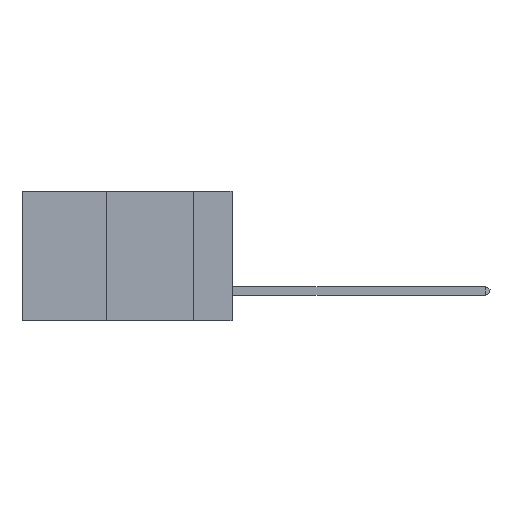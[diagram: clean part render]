
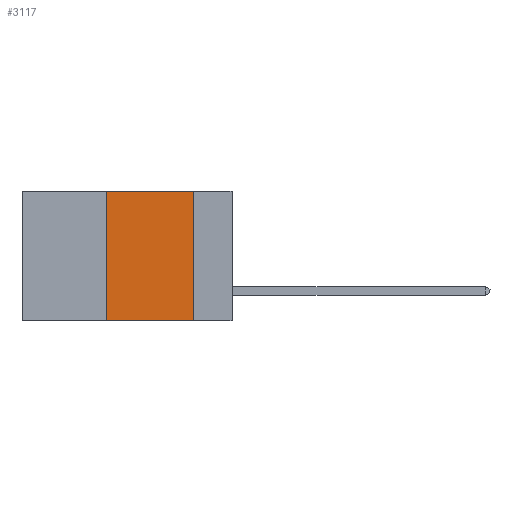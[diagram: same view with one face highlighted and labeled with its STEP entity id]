
A CAD part, left-side view. The second image highlights one B-rep face of the part: STEP entity #3117.
In plain terms, the highlighted planar face has unit normal (-1, 0, 0).
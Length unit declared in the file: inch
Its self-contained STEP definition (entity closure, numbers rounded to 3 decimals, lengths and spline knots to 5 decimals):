
#66 = DIRECTION ( 'NONE',  ( 0., -1., 0. ) ) ;
#553 = EDGE_CURVE ( 'NONE', #4618, #14399, #6563, .T. ) ;
#968 = CARTESIAN_POINT ( 'NONE',  ( 0., 0.36, 0. ) ) ;
#1084 = EDGE_CURVE ( 'NONE', #2751, #14399, #12575, .T. ) ;
#1364 = CARTESIAN_POINT ( 'NONE',  ( 0., 0.6, 0. ) ) ;
#1462 = CARTESIAN_POINT ( 'NONE',  ( 0., 0.6, -0.37 ) ) ;
#1644 = DIRECTION ( 'NONE',  ( 1., 0., 0. ) ) ;
#2654 = FACE_OUTER_BOUND ( 'NONE', #14276, .T. ) ;
#2751 = VERTEX_POINT ( 'NONE', #8409 ) ;
#2947 = ORIENTED_EDGE ( 'NONE', *, *, #553, .T. ) ;
#3117 = ADVANCED_FACE ( 'NONE', ( #2654 ), #6503, .F. ) ;
#3161 = LINE ( 'NONE', #10988, #12844 ) ;
#3299 = ORIENTED_EDGE ( 'NONE', *, *, #1084, .F. ) ;
#4618 = VERTEX_POINT ( 'NONE', #5205 ) ;
#4930 = AXIS2_PLACEMENT_3D ( 'NONE', #5303, #1644, #13589 ) ;
#5205 = CARTESIAN_POINT ( 'NONE',  ( 0., 0.36, -0.37 ) ) ;
#5294 = VERTEX_POINT ( 'NONE', #968 ) ;
#5303 = CARTESIAN_POINT ( 'NONE',  ( 0., 0.6, 0. ) ) ;
#5559 = VECTOR ( 'NONE', #11032, 39.37008 ) ;
#6351 = VECTOR ( 'NONE', #9963, 39.37008 ) ;
#6503 = PLANE ( 'NONE',  #4930 ) ;
#6563 = LINE ( 'NONE', #1462, #6351 ) ;
#7537 = DIRECTION ( 'NONE',  ( 0., 0., 1. ) ) ;
#8409 = CARTESIAN_POINT ( 'NONE',  ( 0., 0.11, 0. ) ) ;
#8515 = LINE ( 'NONE', #1364, #11933 ) ;
#8751 = ORIENTED_EDGE ( 'NONE', *, *, #15065, .F. ) ;
#9497 = CARTESIAN_POINT ( 'NONE',  ( 0., 0.11, -0.37 ) ) ;
#9869 = CARTESIAN_POINT ( 'NONE',  ( 0., 0.11, 0. ) ) ;
#9963 = DIRECTION ( 'NONE',  ( 0., -1., 0. ) ) ;
#10988 = CARTESIAN_POINT ( 'NONE',  ( 0., 0.36, 0. ) ) ;
#11032 = DIRECTION ( 'NONE',  ( 0., 0., -1. ) ) ;
#11491 = ORIENTED_EDGE ( 'NONE', *, *, #15146, .F. ) ;
#11933 = VECTOR ( 'NONE', #66, 39.37008 ) ;
#12575 = LINE ( 'NONE', #9869, #5559 ) ;
#12844 = VECTOR ( 'NONE', #7537, 39.37008 ) ;
#13589 = DIRECTION ( 'NONE',  ( 0., 0., -1. ) ) ;
#14276 = EDGE_LOOP ( 'NONE', ( #3299, #11491, #8751, #2947 ) ) ;
#14399 = VERTEX_POINT ( 'NONE', #9497 ) ;
#15065 = EDGE_CURVE ( 'NONE', #4618, #5294, #3161, .T. ) ;
#15146 = EDGE_CURVE ( 'NONE', #5294, #2751, #8515, .T. ) ;
